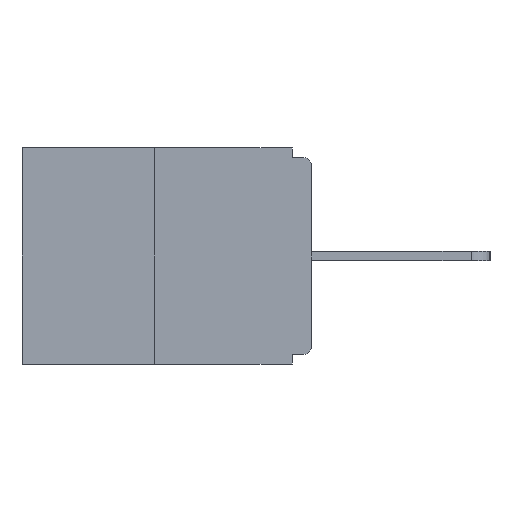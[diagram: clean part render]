
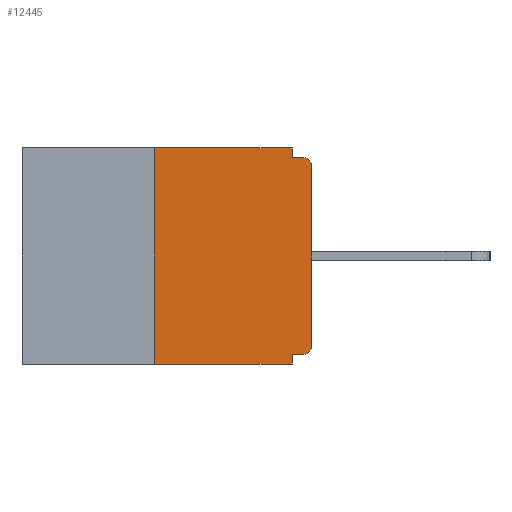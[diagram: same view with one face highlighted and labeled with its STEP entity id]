
A CAD part, left-side view. The second image highlights one B-rep face of the part: STEP entity #12445.
In plain terms, the highlighted planar face has unit normal (-1, 0, 0).
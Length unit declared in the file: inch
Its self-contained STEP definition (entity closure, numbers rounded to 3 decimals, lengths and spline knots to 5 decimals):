
#213 = DIRECTION ( 'NONE',  ( -1., 0., 0. ) ) ;
#671 = DIRECTION ( 'NONE',  ( 0., 0., -1. ) ) ;
#727 = AXIS2_PLACEMENT_3D ( 'NONE', #10398, #213, #5237 ) ;
#803 = ORIENTED_EDGE ( 'NONE', *, *, #2537, .F. ) ;
#952 = VECTOR ( 'NONE', #1491, 39.37008 ) ;
#961 = VECTOR ( 'NONE', #10564, 39.37008 ) ;
#1086 = FACE_OUTER_BOUND ( 'NONE', #7129, .T. ) ;
#1410 = DIRECTION ( 'NONE',  ( 0., -1., 0. ) ) ;
#1491 = DIRECTION ( 'NONE',  ( 0., 0., -1. ) ) ;
#1545 = ORIENTED_EDGE ( 'NONE', *, *, #12139, .T. ) ;
#1596 = EDGE_CURVE ( 'NONE', #7873, #2257, #4340, .T. ) ;
#2148 = PLANE ( 'NONE',  #12062 ) ;
#2257 = VERTEX_POINT ( 'NONE', #8998 ) ;
#2277 = CARTESIAN_POINT ( 'NONE',  ( 0., 0., -0.313 ) ) ;
#2464 = ORIENTED_EDGE ( 'NONE', *, *, #9793, .T. ) ;
#2537 = EDGE_CURVE ( 'NONE', #2693, #12730, #10860, .T. ) ;
#2693 = VERTEX_POINT ( 'NONE', #5082 ) ;
#2759 = LINE ( 'NONE', #4703, #4751 ) ;
#3031 = DIRECTION ( 'NONE',  ( 0., 0., -1. ) ) ;
#3117 = VERTEX_POINT ( 'NONE', #7007 ) ;
#3413 = LINE ( 'NONE', #6487, #7101 ) ;
#3501 = CARTESIAN_POINT ( 'NONE',  ( 0., 0.031, -0.343 ) ) ;
#3752 = ORIENTED_EDGE ( 'NONE', *, *, #5539, .F. ) ;
#3829 = EDGE_CURVE ( 'NONE', #6838, #2693, #2759, .T. ) ;
#3935 = VECTOR ( 'NONE', #9606, 39.37008 ) ;
#4008 = CARTESIAN_POINT ( 'NONE',  ( 0., 0.015, -0.313 ) ) ;
#4231 = CARTESIAN_POINT ( 'NONE',  ( 0., 0.46, 0. ) ) ;
#4340 = LINE ( 'NONE', #12714, #10297 ) ;
#4703 = CARTESIAN_POINT ( 'NONE',  ( 0., 0., -0.328 ) ) ;
#4751 = VECTOR ( 'NONE', #7639, 39.37008 ) ;
#4761 = CARTESIAN_POINT ( 'NONE',  ( 0., 0.031, -0.343 ) ) ;
#4907 = LINE ( 'NONE', #8616, #961 ) ;
#4995 = CIRCLE ( 'NONE', #9492, 0.015 ) ;
#5016 = CARTESIAN_POINT ( 'NONE',  ( 0., 0.25, -0.343 ) ) ;
#5082 = CARTESIAN_POINT ( 'NONE',  ( 0., 0.031, -0.328 ) ) ;
#5110 = ORIENTED_EDGE ( 'NONE', *, *, #11114, .T. ) ;
#5151 = CARTESIAN_POINT ( 'NONE',  ( 0., 0., 0. ) ) ;
#5237 = DIRECTION ( 'NONE',  ( 0., 0., -1. ) ) ;
#5539 = EDGE_CURVE ( 'NONE', #12410, #10872, #4907, .T. ) ;
#5956 = ORIENTED_EDGE ( 'NONE', *, *, #9240, .F. ) ;
#6095 = LINE ( 'NONE', #5151, #11828 ) ;
#6165 = CARTESIAN_POINT ( 'NONE',  ( 0., 0.031, -0.015 ) ) ;
#6270 = DIRECTION ( 'NONE',  ( 0., 0., 1. ) ) ;
#6341 = VECTOR ( 'NONE', #671, 39.37008 ) ;
#6487 = CARTESIAN_POINT ( 'NONE',  ( 0., 0.46, 0. ) ) ;
#6838 = VERTEX_POINT ( 'NONE', #11627 ) ;
#7007 = CARTESIAN_POINT ( 'NONE',  ( 0., 0.031, 0. ) ) ;
#7087 = ORIENTED_EDGE ( 'NONE', *, *, #11604, .T. ) ;
#7101 = VECTOR ( 'NONE', #1410, 39.37008 ) ;
#7129 = EDGE_LOOP ( 'NONE', ( #5956, #11941, #1545, #803, #11467, #2464, #7087, #5110, #3752, #11225 ) ) ;
#7545 = CARTESIAN_POINT ( 'NONE',  ( 0., 0., -0.03 ) ) ;
#7639 = DIRECTION ( 'NONE',  ( 0., 1., 0. ) ) ;
#7705 = DIRECTION ( 'NONE',  ( 0., 0., -1. ) ) ;
#7873 = VERTEX_POINT ( 'NONE', #5016 ) ;
#8012 = VERTEX_POINT ( 'NONE', #7545 ) ;
#8200 = CARTESIAN_POINT ( 'NONE',  ( 0., 0.031, 0. ) ) ;
#8332 = LINE ( 'NONE', #8200, #952 ) ;
#8616 = CARTESIAN_POINT ( 'NONE',  ( 0., 0., -0.015 ) ) ;
#8998 = CARTESIAN_POINT ( 'NONE',  ( 0., 0.25, 0. ) ) ;
#9240 = EDGE_CURVE ( 'NONE', #2257, #3117, #3413, .T. ) ;
#9264 = DIRECTION ( 'NONE',  ( 1., 0., 0. ) ) ;
#9492 = AXIS2_PLACEMENT_3D ( 'NONE', #4008, #12944, #7705 ) ;
#9606 = DIRECTION ( 'NONE',  ( 0., -1., 0. ) ) ;
#9793 = EDGE_CURVE ( 'NONE', #6838, #11763, #4995, .T. ) ;
#10191 = DIRECTION ( 'NONE',  ( 0., 0., 1. ) ) ;
#10297 = VECTOR ( 'NONE', #6270, 39.37008 ) ;
#10398 = CARTESIAN_POINT ( 'NONE',  ( 0., 0.015, -0.03 ) ) ;
#10564 = DIRECTION ( 'NONE',  ( 0., -1., 0. ) ) ;
#10811 = LINE ( 'NONE', #11805, #3935 ) ;
#10813 = EDGE_CURVE ( 'NONE', #3117, #12410, #8332, .T. ) ;
#10860 = LINE ( 'NONE', #3501, #6341 ) ;
#10872 = VERTEX_POINT ( 'NONE', #12614 ) ;
#11114 = EDGE_CURVE ( 'NONE', #8012, #10872, #11644, .T. ) ;
#11225 = ORIENTED_EDGE ( 'NONE', *, *, #10813, .F. ) ;
#11467 = ORIENTED_EDGE ( 'NONE', *, *, #3829, .F. ) ;
#11604 = EDGE_CURVE ( 'NONE', #11763, #8012, #6095, .T. ) ;
#11627 = CARTESIAN_POINT ( 'NONE',  ( 0., 0.015, -0.328 ) ) ;
#11644 = CIRCLE ( 'NONE', #727, 0.015 ) ;
#11763 = VERTEX_POINT ( 'NONE', #2277 ) ;
#11805 = CARTESIAN_POINT ( 'NONE',  ( 0., 0.46, -0.343 ) ) ;
#11828 = VECTOR ( 'NONE', #10191, 39.37008 ) ;
#11941 = ORIENTED_EDGE ( 'NONE', *, *, #1596, .F. ) ;
#12062 = AXIS2_PLACEMENT_3D ( 'NONE', #4231, #9264, #3031 ) ;
#12139 = EDGE_CURVE ( 'NONE', #7873, #12730, #10811, .T. ) ;
#12410 = VERTEX_POINT ( 'NONE', #6165 ) ;
#12445 = ADVANCED_FACE ( 'NONE', ( #1086 ), #2148, .F. ) ;
#12614 = CARTESIAN_POINT ( 'NONE',  ( 0., 0.015, -0.015 ) ) ;
#12714 = CARTESIAN_POINT ( 'NONE',  ( 0., 0.25, 0. ) ) ;
#12730 = VERTEX_POINT ( 'NONE', #4761 ) ;
#12944 = DIRECTION ( 'NONE',  ( -1., 0., 0. ) ) ;
